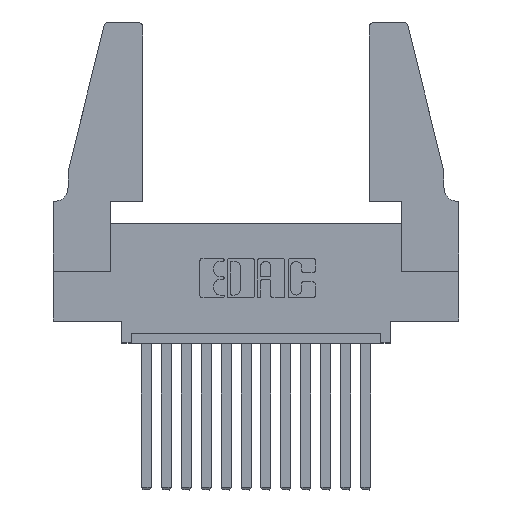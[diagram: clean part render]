
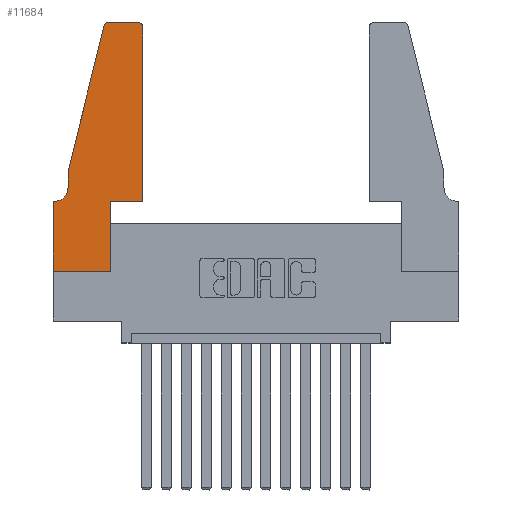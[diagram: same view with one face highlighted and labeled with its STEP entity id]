
A CAD part, top view. The second image highlights one B-rep face of the part: STEP entity #11684.
In plain terms, the highlighted planar face has unit normal (0, 0, 1).
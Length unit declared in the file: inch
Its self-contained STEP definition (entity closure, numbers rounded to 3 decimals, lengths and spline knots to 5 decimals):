
#6 = CARTESIAN_POINT ( 'NONE',  ( 0.2605, 1.25, 0.37 ) ) ;
#434 = LINE ( 'NONE', #6, #985 ) ;
#506 = CARTESIAN_POINT ( 'NONE',  ( 0., 0.35, 0.37 ) ) ;
#640 = EDGE_CURVE ( 'NONE', #8654, #8093, #12323, .T. ) ;
#746 = CARTESIAN_POINT ( 'NONE',  ( 0.0755, 0.5, 0.37 ) ) ;
#985 = VECTOR ( 'NONE', #7199, 39.37008 ) ;
#991 = ORIENTED_EDGE ( 'NONE', *, *, #1957, .T. ) ;
#1206 = CARTESIAN_POINT ( 'NONE',  ( 0., 0., 0.37 ) ) ;
#1245 = VECTOR ( 'NONE', #6555, 39.37008 ) ;
#1606 = VERTEX_POINT ( 'NONE', #6021 ) ;
#1614 = DIRECTION ( 'NONE',  ( 0., 1., 0. ) ) ;
#1693 = VECTOR ( 'NONE', #1614, 39.37008 ) ;
#1842 = CARTESIAN_POINT ( 'NONE',  ( 0.284, 1.22, 0.37 ) ) ;
#1957 = EDGE_CURVE ( 'NONE', #11667, #8654, #13187, .T. ) ;
#2062 = VECTOR ( 'NONE', #12137, 39.37008 ) ;
#2111 = VERTEX_POINT ( 'NONE', #4917 ) ;
#2182 = LINE ( 'NONE', #746, #5665 ) ;
#2358 = LINE ( 'NONE', #11212, #5303 ) ;
#2401 = CARTESIAN_POINT ( 'NONE',  ( 0.4505, 0.35, 0.37 ) ) ;
#2547 = ORIENTED_EDGE ( 'NONE', *, *, #7354, .T. ) ;
#2566 = VERTEX_POINT ( 'NONE', #506 ) ;
#2672 = EDGE_LOOP ( 'NONE', ( #5916, #10991, #5868, #13827, #10635, #6241, #2743, #6227, #9943, #991, #11972, #2547 ) ) ;
#2743 = ORIENTED_EDGE ( 'NONE', *, *, #5775, .T. ) ;
#3032 = DIRECTION ( 'NONE',  ( 1., 0., 0. ) ) ;
#3387 = CIRCLE ( 'NONE', #4391, 0.03 ) ;
#3437 = CIRCLE ( 'NONE', #10166, 0.03 ) ;
#3557 = DIRECTION ( 'NONE',  ( 0., 0., -1. ) ) ;
#3671 = CARTESIAN_POINT ( 'NONE',  ( 0.4205, 1.25, 0.37 ) ) ;
#4093 = CARTESIAN_POINT ( 'NONE',  ( 0.4505, 0.35, 0.37 ) ) ;
#4391 = AXIS2_PLACEMENT_3D ( 'NONE', #1842, #12464, #3032 ) ;
#4607 = VERTEX_POINT ( 'NONE', #14020 ) ;
#4917 = CARTESIAN_POINT ( 'NONE',  ( 0.25487, 1.22718, 0.37 ) ) ;
#4965 = EDGE_CURVE ( 'NONE', #12099, #1606, #434, .T. ) ;
#5139 = FACE_OUTER_BOUND ( 'NONE', #2672, .T. ) ;
#5303 = VECTOR ( 'NONE', #6495, 39.37008 ) ;
#5551 = LINE ( 'NONE', #14479, #1693 ) ;
#5585 = AXIS2_PLACEMENT_3D ( 'NONE', #10096, #6458, #7630 ) ;
#5665 = VECTOR ( 'NONE', #13504, 39.37008 ) ;
#5752 = VERTEX_POINT ( 'NONE', #13992 ) ;
#5775 = EDGE_CURVE ( 'NONE', #2566, #7756, #7017, .T. ) ;
#5868 = ORIENTED_EDGE ( 'NONE', *, *, #13026, .T. ) ;
#5916 = ORIENTED_EDGE ( 'NONE', *, *, #4965, .T. ) ;
#6021 = CARTESIAN_POINT ( 'NONE',  ( 0.284, 1.25, 0.37 ) ) ;
#6022 = LINE ( 'NONE', #14742, #1245 ) ;
#6227 = ORIENTED_EDGE ( 'NONE', *, *, #12382, .T. ) ;
#6241 = ORIENTED_EDGE ( 'NONE', *, *, #12441, .T. ) ;
#6458 = DIRECTION ( 'NONE',  ( 0., 0., 1. ) ) ;
#6495 = DIRECTION ( 'NONE',  ( 1., 0., 0. ) ) ;
#6534 = CARTESIAN_POINT ( 'NONE',  ( 0.4205, 1.22, 0.37 ) ) ;
#6555 = DIRECTION ( 'NONE',  ( -0.239, -0.971, 0. ) ) ;
#7017 = LINE ( 'NONE', #1206, #12513 ) ;
#7199 = DIRECTION ( 'NONE',  ( -1., 0., 0. ) ) ;
#7354 = EDGE_CURVE ( 'NONE', #8093, #12099, #3437, .T. ) ;
#7630 = DIRECTION ( 'NONE',  ( 1., 0., 0. ) ) ;
#7756 = VERTEX_POINT ( 'NONE', #10731 ) ;
#8093 = VERTEX_POINT ( 'NONE', #9773 ) ;
#8431 = DIRECTION ( 'NONE',  ( 0., -1., 0. ) ) ;
#8654 = VERTEX_POINT ( 'NONE', #9369 ) ;
#9369 = CARTESIAN_POINT ( 'NONE',  ( 0.4505, 0.35, 0.37 ) ) ;
#9646 = EDGE_CURVE ( 'NONE', #1606, #2111, #3387, .T. ) ;
#9735 = VERTEX_POINT ( 'NONE', #11557 ) ;
#9773 = CARTESIAN_POINT ( 'NONE',  ( 0.4505, 1.22, 0.37 ) ) ;
#9943 = ORIENTED_EDGE ( 'NONE', *, *, #13682, .T. ) ;
#10082 = VECTOR ( 'NONE', #15166, 39.37008 ) ;
#10096 = CARTESIAN_POINT ( 'NONE',  ( 0., 0.35, 0.37 ) ) ;
#10166 = AXIS2_PLACEMENT_3D ( 'NONE', #6534, #11254, #11206 ) ;
#10393 = AXIS2_PLACEMENT_3D ( 'NONE', #10582, #3557, #12985 ) ;
#10442 = VECTOR ( 'NONE', #14628, 39.37008 ) ;
#10582 = CARTESIAN_POINT ( 'NONE',  ( 0.0055, 0.42, 0.37 ) ) ;
#10635 = ORIENTED_EDGE ( 'NONE', *, *, #10928, .T. ) ;
#10731 = CARTESIAN_POINT ( 'NONE',  ( 0., 0., 0.37 ) ) ;
#10846 = CIRCLE ( 'NONE', #10393, 0.07 ) ;
#10928 = EDGE_CURVE ( 'NONE', #11349, #5752, #10846, .T. ) ;
#10991 = ORIENTED_EDGE ( 'NONE', *, *, #9646, .T. ) ;
#11133 = CARTESIAN_POINT ( 'NONE',  ( 0.2865, 0.35, 0.37 ) ) ;
#11206 = DIRECTION ( 'NONE',  ( 1., 0., 0. ) ) ;
#11212 = CARTESIAN_POINT ( 'NONE',  ( 0., 0., 0.37 ) ) ;
#11254 = DIRECTION ( 'NONE',  ( 0., 0., 1. ) ) ;
#11349 = VERTEX_POINT ( 'NONE', #11712 ) ;
#11557 = CARTESIAN_POINT ( 'NONE',  ( 0.2865, 0., 0.37 ) ) ;
#11667 = VERTEX_POINT ( 'NONE', #11133 ) ;
#11684 = ADVANCED_FACE ( 'NONE', ( #5139 ), #13467, .T. ) ;
#11712 = CARTESIAN_POINT ( 'NONE',  ( 0.0755, 0.42, 0.37 ) ) ;
#11972 = ORIENTED_EDGE ( 'NONE', *, *, #640, .T. ) ;
#12099 = VERTEX_POINT ( 'NONE', #3671 ) ;
#12137 = DIRECTION ( 'NONE',  ( 0., 1., 0. ) ) ;
#12323 = LINE ( 'NONE', #4093, #2062 ) ;
#12382 = EDGE_CURVE ( 'NONE', #7756, #9735, #2358, .T. ) ;
#12389 = CARTESIAN_POINT ( 'NONE',  ( 0.0755, 0.35, 0.37 ) ) ;
#12408 = EDGE_CURVE ( 'NONE', #4607, #11349, #2182, .T. ) ;
#12441 = EDGE_CURVE ( 'NONE', #5752, #2566, #14283, .T. ) ;
#12464 = DIRECTION ( 'NONE',  ( 0., 0., 1. ) ) ;
#12513 = VECTOR ( 'NONE', #8431, 39.37008 ) ;
#12985 = DIRECTION ( 'NONE',  ( -1., 0., 0. ) ) ;
#13026 = EDGE_CURVE ( 'NONE', #2111, #4607, #6022, .T. ) ;
#13187 = LINE ( 'NONE', #2401, #10082 ) ;
#13467 = PLANE ( 'NONE',  #5585 ) ;
#13504 = DIRECTION ( 'NONE',  ( 0., -1., 0. ) ) ;
#13682 = EDGE_CURVE ( 'NONE', #9735, #11667, #5551, .T. ) ;
#13827 = ORIENTED_EDGE ( 'NONE', *, *, #12408, .T. ) ;
#13992 = CARTESIAN_POINT ( 'NONE',  ( 0.0055, 0.35, 0.37 ) ) ;
#14020 = CARTESIAN_POINT ( 'NONE',  ( 0.0755, 0.5, 0.37 ) ) ;
#14283 = LINE ( 'NONE', #12389, #10442 ) ;
#14479 = CARTESIAN_POINT ( 'NONE',  ( 0.2865, 0.35, 0.37 ) ) ;
#14628 = DIRECTION ( 'NONE',  ( -1., 0., 0. ) ) ;
#14742 = CARTESIAN_POINT ( 'NONE',  ( 0.0755, 0.5, 0.37 ) ) ;
#15166 = DIRECTION ( 'NONE',  ( 1., 0., 0. ) ) ;
